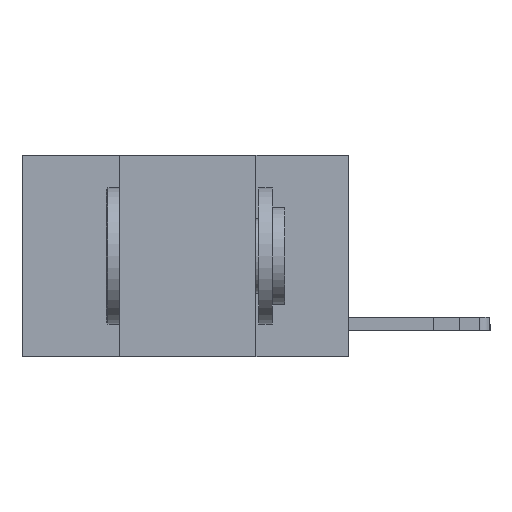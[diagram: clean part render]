
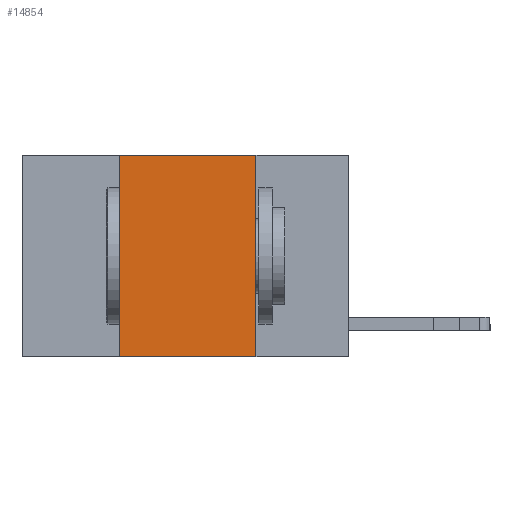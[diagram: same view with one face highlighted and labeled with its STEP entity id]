
A CAD part, left-side view. The second image highlights one B-rep face of the part: STEP entity #14854.
In plain terms, the highlighted planar face has unit normal (-1, 0, 0).
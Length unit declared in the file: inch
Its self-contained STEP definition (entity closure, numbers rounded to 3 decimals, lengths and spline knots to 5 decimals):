
#402 = EDGE_CURVE ( 'NONE', #5180, #14417, #13485, .T. ) ;
#686 = EDGE_CURVE ( 'NONE', #14417, #12327, #3398, .T. ) ;
#1320 = ORIENTED_EDGE ( 'NONE', *, *, #14228, .F. ) ;
#1445 = VECTOR ( 'NONE', #11123, 39.37008 ) ;
#1489 = CARTESIAN_POINT ( 'NONE',  ( 0., 0.17, -0.37 ) ) ;
#1821 = CARTESIAN_POINT ( 'NONE',  ( 0., 0.42, 0. ) ) ;
#3052 = DIRECTION ( 'NONE',  ( 0., 0., 1. ) ) ;
#3398 = LINE ( 'NONE', #8352, #7630 ) ;
#3600 = CARTESIAN_POINT ( 'NONE',  ( 0., 0.6, 0. ) ) ;
#4401 = LINE ( 'NONE', #13346, #9061 ) ;
#4777 = ORIENTED_EDGE ( 'NONE', *, *, #402, .F. ) ;
#4987 = VERTEX_POINT ( 'NONE', #6616 ) ;
#5180 = VERTEX_POINT ( 'NONE', #1821 ) ;
#6317 = CARTESIAN_POINT ( 'NONE',  ( 0., 0.17, 0. ) ) ;
#6351 = LINE ( 'NONE', #7945, #6500 ) ;
#6500 = VECTOR ( 'NONE', #11371, 39.37008 ) ;
#6616 = CARTESIAN_POINT ( 'NONE',  ( 0., 0.42, -0.37 ) ) ;
#6764 = EDGE_CURVE ( 'NONE', #4987, #12327, #6351, .T. ) ;
#7020 = DIRECTION ( 'NONE',  ( 0., 0., -1. ) ) ;
#7630 = VECTOR ( 'NONE', #7020, 39.37008 ) ;
#7641 = DIRECTION ( 'NONE',  ( 0., 0., -1. ) ) ;
#7945 = CARTESIAN_POINT ( 'NONE',  ( 0., 0.6, -0.37 ) ) ;
#8352 = CARTESIAN_POINT ( 'NONE',  ( 0., 0.17, 0. ) ) ;
#8782 = AXIS2_PLACEMENT_3D ( 'NONE', #3600, #12730, #7641 ) ;
#9061 = VECTOR ( 'NONE', #3052, 39.37008 ) ;
#11123 = DIRECTION ( 'NONE',  ( 0., -1., 0. ) ) ;
#11167 = ORIENTED_EDGE ( 'NONE', *, *, #6764, .T. ) ;
#11371 = DIRECTION ( 'NONE',  ( 0., -1., 0. ) ) ;
#11566 = PLANE ( 'NONE',  #8782 ) ;
#12327 = VERTEX_POINT ( 'NONE', #1489 ) ;
#12730 = DIRECTION ( 'NONE',  ( 1., 0., 0. ) ) ;
#13346 = CARTESIAN_POINT ( 'NONE',  ( 0., 0.42, 0. ) ) ;
#13485 = LINE ( 'NONE', #14741, #1445 ) ;
#14228 = EDGE_CURVE ( 'NONE', #4987, #5180, #4401, .T. ) ;
#14417 = VERTEX_POINT ( 'NONE', #6317 ) ;
#14741 = CARTESIAN_POINT ( 'NONE',  ( 0., 0.6, 0. ) ) ;
#14854 = ADVANCED_FACE ( 'NONE', ( #15174 ), #11566, .F. ) ;
#15076 = EDGE_LOOP ( 'NONE', ( #16407, #4777, #1320, #11167 ) ) ;
#15174 = FACE_OUTER_BOUND ( 'NONE', #15076, .T. ) ;
#16407 = ORIENTED_EDGE ( 'NONE', *, *, #686, .F. ) ;
